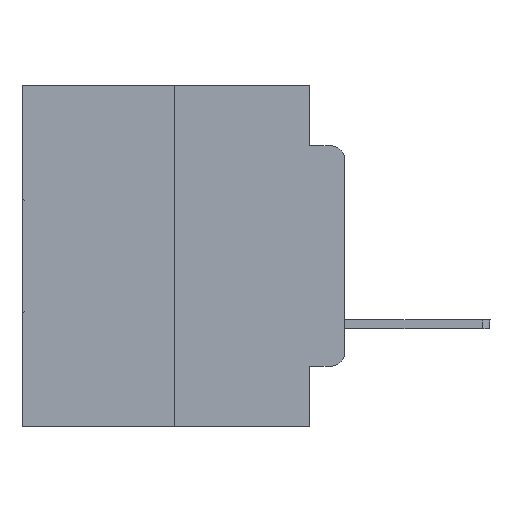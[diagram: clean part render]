
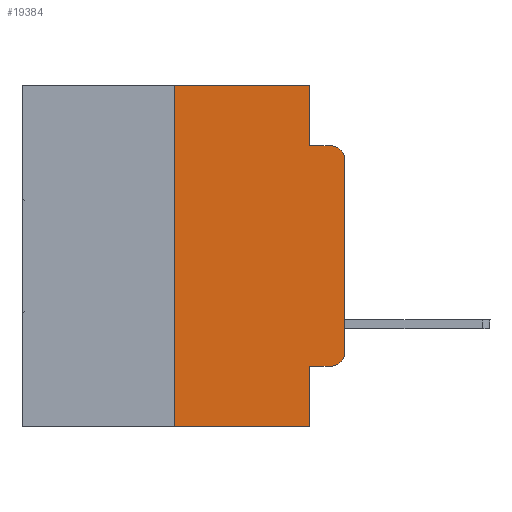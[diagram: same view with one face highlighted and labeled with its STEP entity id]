
A CAD part, left-side view. The second image highlights one B-rep face of the part: STEP entity #19384.
In plain terms, the highlighted planar face has unit normal (-1, 0, 0).
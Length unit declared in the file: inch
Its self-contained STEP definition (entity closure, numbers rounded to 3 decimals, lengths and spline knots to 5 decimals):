
#31 = CARTESIAN_POINT ( 'NONE',  ( 0., 0.02, -0.3915 ) ) ;
#953 = DIRECTION ( 'NONE',  ( 0., 0., -1. ) ) ;
#1031 = PLANE ( 'NONE',  #2431 ) ;
#1032 = AXIS2_PLACEMENT_3D ( 'NONE', #31, #9009, #18126 ) ;
#2431 = AXIS2_PLACEMENT_3D ( 'NONE', #27213, #19415, #25725 ) ;
#2708 = VECTOR ( 'NONE', #11755, 39.37008 ) ;
#3356 = VECTOR ( 'NONE', #14816, 39.37008 ) ;
#4347 = VECTOR ( 'NONE', #22427, 39.37008 ) ;
#4495 = LINE ( 'NONE', #10647, #4347 ) ;
#4760 = VECTOR ( 'NONE', #14607, 39.37008 ) ;
#5308 = ORIENTED_EDGE ( 'NONE', *, *, #6332, .F. ) ;
#5348 = VERTEX_POINT ( 'NONE', #10645 ) ;
#5931 = CARTESIAN_POINT ( 'NONE',  ( 0., 0.051, 0. ) ) ;
#6072 = DIRECTION ( 'NONE',  ( 0., 0., -1. ) ) ;
#6332 = EDGE_CURVE ( 'NONE', #5348, #20334, #15874, .T. ) ;
#6613 = CARTESIAN_POINT ( 'NONE',  ( 0., 0.25, 0. ) ) ;
#8396 = CIRCLE ( 'NONE', #14507, 0.02 ) ;
#8943 = EDGE_LOOP ( 'NONE', ( #13209, #21658, #27870, #19264, #26109, #21992, #12589, #5308, #18690, #19500 ) ) ;
#9009 = DIRECTION ( 'NONE',  ( -1., 0., 0. ) ) ;
#9965 = LINE ( 'NONE', #12168, #3356 ) ;
#10331 = EDGE_CURVE ( 'NONE', #23175, #22372, #9965, .T. ) ;
#10645 = CARTESIAN_POINT ( 'NONE',  ( 0., 0.051, -0.4115 ) ) ;
#10647 = CARTESIAN_POINT ( 'NONE',  ( 0., 0.051, -0.4115 ) ) ;
#10820 = VERTEX_POINT ( 'NONE', #13012 ) ;
#11141 = EDGE_CURVE ( 'NONE', #27661, #26919, #16520, .T. ) ;
#11755 = DIRECTION ( 'NONE',  ( 0., 0., -1. ) ) ;
#12168 = CARTESIAN_POINT ( 'NONE',  ( 0., 0.051, -0.0885 ) ) ;
#12307 = CIRCLE ( 'NONE', #1032, 0.02 ) ;
#12589 = ORIENTED_EDGE ( 'NONE', *, *, #24928, .T. ) ;
#12688 = CARTESIAN_POINT ( 'NONE',  ( 0., 0.051, 0. ) ) ;
#12780 = EDGE_CURVE ( 'NONE', #22436, #25123, #12307, .T. ) ;
#13012 = CARTESIAN_POINT ( 'NONE',  ( 0., 0., -0.1085 ) ) ;
#13209 = ORIENTED_EDGE ( 'NONE', *, *, #27788, .T. ) ;
#13801 = EDGE_CURVE ( 'NONE', #28950, #27661, #28788, .T. ) ;
#14016 = CARTESIAN_POINT ( 'NONE',  ( 0., 0.02, -0.0885 ) ) ;
#14255 = CARTESIAN_POINT ( 'NONE',  ( 0., 0.25, 0. ) ) ;
#14507 = AXIS2_PLACEMENT_3D ( 'NONE', #18479, #21109, #953 ) ;
#14607 = DIRECTION ( 'NONE',  ( 0., -1., 0. ) ) ;
#14816 = DIRECTION ( 'NONE',  ( 0., -1., 0. ) ) ;
#15582 = DIRECTION ( 'NONE',  ( 0., 0., 1. ) ) ;
#15874 = LINE ( 'NONE', #16022, #2708 ) ;
#16022 = CARTESIAN_POINT ( 'NONE',  ( 0., 0.051, 0. ) ) ;
#16520 = LINE ( 'NONE', #27529, #4760 ) ;
#16743 = CARTESIAN_POINT ( 'NONE',  ( 0., 0.25, -0.5 ) ) ;
#17120 = EDGE_CURVE ( 'NONE', #10820, #22372, #8396, .T. ) ;
#17912 = DIRECTION ( 'NONE',  ( 0., -1., 0. ) ) ;
#18126 = DIRECTION ( 'NONE',  ( 0., 0., -1. ) ) ;
#18378 = CARTESIAN_POINT ( 'NONE',  ( 0., 0.051, -0.0885 ) ) ;
#18479 = CARTESIAN_POINT ( 'NONE',  ( 0., 0.02, -0.1085 ) ) ;
#18690 = ORIENTED_EDGE ( 'NONE', *, *, #20488, .T. ) ;
#19239 = LINE ( 'NONE', #21747, #23398 ) ;
#19264 = ORIENTED_EDGE ( 'NONE', *, *, #20854, .F. ) ;
#19384 = ADVANCED_FACE ( 'NONE', ( #21188 ), #1031, .F. ) ;
#19415 = DIRECTION ( 'NONE',  ( 1., 0., 0. ) ) ;
#19500 = ORIENTED_EDGE ( 'NONE', *, *, #12780, .T. ) ;
#19788 = VECTOR ( 'NONE', #6072, 39.37008 ) ;
#20121 = LINE ( 'NONE', #29051, #24225 ) ;
#20334 = VERTEX_POINT ( 'NONE', #27855 ) ;
#20488 = EDGE_CURVE ( 'NONE', #5348, #22436, #4495, .T. ) ;
#20854 = EDGE_CURVE ( 'NONE', #26919, #23175, #26785, .T. ) ;
#21109 = DIRECTION ( 'NONE',  ( -1., 0., 0. ) ) ;
#21188 = FACE_OUTER_BOUND ( 'NONE', #8943, .T. ) ;
#21658 = ORIENTED_EDGE ( 'NONE', *, *, #17120, .T. ) ;
#21747 = CARTESIAN_POINT ( 'NONE',  ( 0., 0., 0. ) ) ;
#21992 = ORIENTED_EDGE ( 'NONE', *, *, #13801, .F. ) ;
#22372 = VERTEX_POINT ( 'NONE', #14016 ) ;
#22427 = DIRECTION ( 'NONE',  ( 0., -1., 0. ) ) ;
#22436 = VERTEX_POINT ( 'NONE', #25915 ) ;
#23175 = VERTEX_POINT ( 'NONE', #18378 ) ;
#23398 = VECTOR ( 'NONE', #26288, 39.37008 ) ;
#24225 = VECTOR ( 'NONE', #17912, 39.37008 ) ;
#24928 = EDGE_CURVE ( 'NONE', #28950, #20334, #20121, .T. ) ;
#25055 = CARTESIAN_POINT ( 'NONE',  ( 0., 0., -0.3915 ) ) ;
#25123 = VERTEX_POINT ( 'NONE', #25055 ) ;
#25725 = DIRECTION ( 'NONE',  ( 0., 0., -1. ) ) ;
#25915 = CARTESIAN_POINT ( 'NONE',  ( 0., 0.02, -0.4115 ) ) ;
#26109 = ORIENTED_EDGE ( 'NONE', *, *, #11141, .F. ) ;
#26288 = DIRECTION ( 'NONE',  ( 0., 0., 1. ) ) ;
#26785 = LINE ( 'NONE', #12688, #19788 ) ;
#26919 = VERTEX_POINT ( 'NONE', #5931 ) ;
#27213 = CARTESIAN_POINT ( 'NONE',  ( 0., 0.473, 0. ) ) ;
#27529 = CARTESIAN_POINT ( 'NONE',  ( 0., 0.473, 0. ) ) ;
#27661 = VERTEX_POINT ( 'NONE', #14255 ) ;
#27788 = EDGE_CURVE ( 'NONE', #25123, #10820, #19239, .T. ) ;
#27855 = CARTESIAN_POINT ( 'NONE',  ( 0., 0.051, -0.5 ) ) ;
#27870 = ORIENTED_EDGE ( 'NONE', *, *, #10331, .F. ) ;
#28302 = VECTOR ( 'NONE', #15582, 39.37008 ) ;
#28788 = LINE ( 'NONE', #6613, #28302 ) ;
#28950 = VERTEX_POINT ( 'NONE', #16743 ) ;
#29051 = CARTESIAN_POINT ( 'NONE',  ( 0., 0.473, -0.5 ) ) ;
